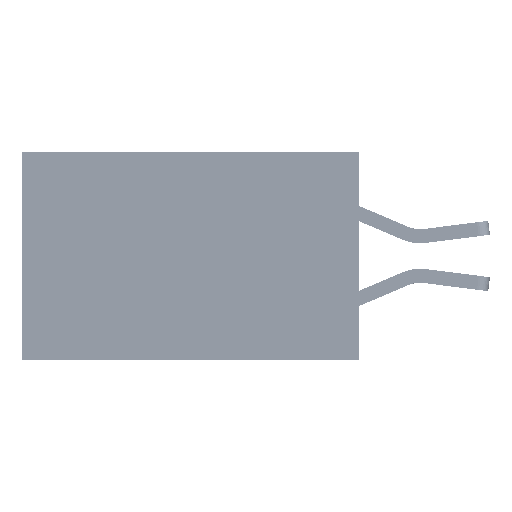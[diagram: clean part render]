
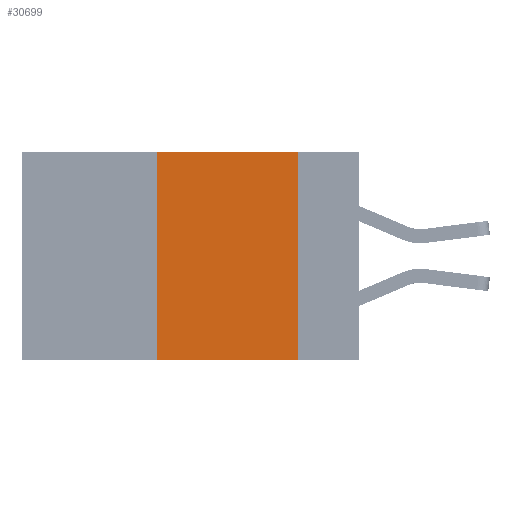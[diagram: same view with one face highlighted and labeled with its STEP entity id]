
A CAD part, left-side view. The second image highlights one B-rep face of the part: STEP entity #30699.
In plain terms, the highlighted planar face has unit normal (-1, 0, 0).
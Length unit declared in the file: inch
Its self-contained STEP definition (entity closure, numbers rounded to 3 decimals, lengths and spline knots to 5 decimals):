
#1448 = VECTOR ( 'NONE', #41967, 39.37008 ) ;
#3607 = CARTESIAN_POINT ( 'NONE',  ( 0., 0.6, 0. ) ) ;
#3834 = LINE ( 'NONE', #3607, #35081 ) ;
#3860 = ORIENTED_EDGE ( 'NONE', *, *, #31247, .F. ) ;
#6019 = CARTESIAN_POINT ( 'NONE',  ( 0., 0.36, 0. ) ) ;
#6272 = CARTESIAN_POINT ( 'NONE',  ( 0., 0.6, 0. ) ) ;
#6576 = VECTOR ( 'NONE', #26903, 39.37008 ) ;
#7957 = VERTEX_POINT ( 'NONE', #30909 ) ;
#8219 = CARTESIAN_POINT ( 'NONE',  ( 0., 0.36, -0.37 ) ) ;
#8468 = AXIS2_PLACEMENT_3D ( 'NONE', #6272, #34226, #38202 ) ;
#9986 = LINE ( 'NONE', #35734, #21817 ) ;
#11861 = DIRECTION ( 'NONE',  ( 0., -1., 0. ) ) ;
#15325 = ORIENTED_EDGE ( 'NONE', *, *, #15476, .F. ) ;
#15476 = EDGE_CURVE ( 'NONE', #29439, #7957, #25878, .T. ) ;
#15830 = LINE ( 'NONE', #6019, #1448 ) ;
#20630 = EDGE_CURVE ( 'NONE', #40027, #43367, #15830, .T. ) ;
#20831 = CARTESIAN_POINT ( 'NONE',  ( 0., 0.36, 0. ) ) ;
#21817 = VECTOR ( 'NONE', #11861, 39.37008 ) ;
#22145 = PLANE ( 'NONE',  #8468 ) ;
#24225 = ORIENTED_EDGE ( 'NONE', *, *, #20630, .F. ) ;
#25878 = LINE ( 'NONE', #50657, #6576 ) ;
#26903 = DIRECTION ( 'NONE',  ( 0., 0., -1. ) ) ;
#29439 = VERTEX_POINT ( 'NONE', #49828 ) ;
#30699 = ADVANCED_FACE ( 'NONE', ( #51323 ), #22145, .F. ) ;
#30909 = CARTESIAN_POINT ( 'NONE',  ( 0., 0.11, -0.37 ) ) ;
#30985 = EDGE_LOOP ( 'NONE', ( #15325, #3860, #24225, #48907 ) ) ;
#31247 = EDGE_CURVE ( 'NONE', #43367, #29439, #3834, .T. ) ;
#34226 = DIRECTION ( 'NONE',  ( 1., 0., 0. ) ) ;
#35081 = VECTOR ( 'NONE', #35537, 39.37008 ) ;
#35537 = DIRECTION ( 'NONE',  ( 0., -1., 0. ) ) ;
#35734 = CARTESIAN_POINT ( 'NONE',  ( 0., 0.6, -0.37 ) ) ;
#38202 = DIRECTION ( 'NONE',  ( 0., 0., -1. ) ) ;
#40027 = VERTEX_POINT ( 'NONE', #8219 ) ;
#41225 = EDGE_CURVE ( 'NONE', #40027, #7957, #9986, .T. ) ;
#41967 = DIRECTION ( 'NONE',  ( 0., 0., 1. ) ) ;
#43367 = VERTEX_POINT ( 'NONE', #20831 ) ;
#48907 = ORIENTED_EDGE ( 'NONE', *, *, #41225, .T. ) ;
#49828 = CARTESIAN_POINT ( 'NONE',  ( 0., 0.11, 0. ) ) ;
#50657 = CARTESIAN_POINT ( 'NONE',  ( 0., 0.11, 0. ) ) ;
#51323 = FACE_OUTER_BOUND ( 'NONE', #30985, .T. ) ;
